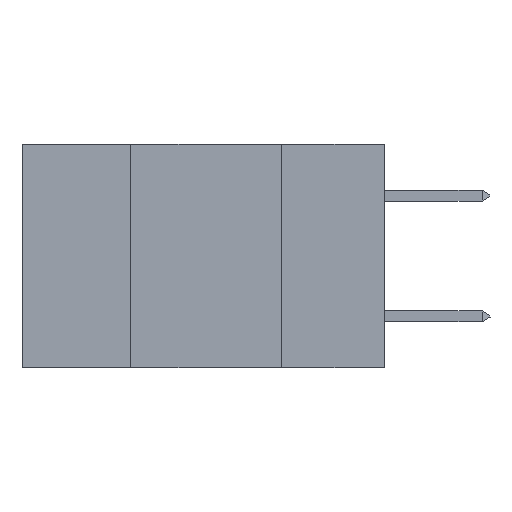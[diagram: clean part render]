
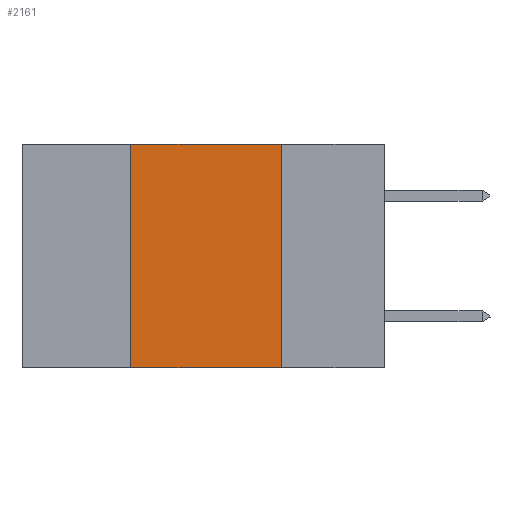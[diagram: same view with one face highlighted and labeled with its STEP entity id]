
A CAD part, left-side view. The second image highlights one B-rep face of the part: STEP entity #2161.
In plain terms, the highlighted planar face has unit normal (-1, 0, 0).
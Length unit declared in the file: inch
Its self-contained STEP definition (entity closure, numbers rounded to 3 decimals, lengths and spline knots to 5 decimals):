
#735 = VERTEX_POINT ( 'NONE', #7544 ) ;
#887 = CARTESIAN_POINT ( 'NONE',  ( 0., 0.42, -0.37 ) ) ;
#976 = VECTOR ( 'NONE', #5215, 39.37008 ) ;
#1231 = VERTEX_POINT ( 'NONE', #7557 ) ;
#1275 = VECTOR ( 'NONE', #4419, 39.37008 ) ;
#1786 = EDGE_LOOP ( 'NONE', ( #6654, #8103, #6742, #5730 ) ) ;
#2161 = ADVANCED_FACE ( 'NONE', ( #8982 ), #8652, .F. ) ;
#2275 = CARTESIAN_POINT ( 'NONE',  ( 0., 0.42, 0. ) ) ;
#2564 = EDGE_CURVE ( 'NONE', #8297, #735, #4637, .T. ) ;
#2744 = EDGE_CURVE ( 'NONE', #1231, #7260, #3077, .T. ) ;
#2819 = CARTESIAN_POINT ( 'NONE',  ( 0., 0.17, 0. ) ) ;
#2945 = DIRECTION ( 'NONE',  ( 0., 0., 1. ) ) ;
#3077 = LINE ( 'NONE', #4408, #1275 ) ;
#3910 = CARTESIAN_POINT ( 'NONE',  ( 0., 0.17, 0. ) ) ;
#4101 = CARTESIAN_POINT ( 'NONE',  ( 0., 0.6, -0.37 ) ) ;
#4186 = VECTOR ( 'NONE', #6700, 39.37008 ) ;
#4408 = CARTESIAN_POINT ( 'NONE',  ( 0., 0.6, 0. ) ) ;
#4419 = DIRECTION ( 'NONE',  ( 0., -1., 0. ) ) ;
#4572 = LINE ( 'NONE', #2275, #8159 ) ;
#4637 = LINE ( 'NONE', #4101, #4186 ) ;
#5215 = DIRECTION ( 'NONE',  ( 0., 0., -1. ) ) ;
#5413 = DIRECTION ( 'NONE',  ( 1., 0., 0. ) ) ;
#5577 = CARTESIAN_POINT ( 'NONE',  ( 0., 0.6, 0. ) ) ;
#5730 = ORIENTED_EDGE ( 'NONE', *, *, #2564, .T. ) ;
#5745 = EDGE_CURVE ( 'NONE', #7260, #735, #6426, .T. ) ;
#5927 = DIRECTION ( 'NONE',  ( 0., 0., -1. ) ) ;
#6426 = LINE ( 'NONE', #3910, #976 ) ;
#6654 = ORIENTED_EDGE ( 'NONE', *, *, #5745, .F. ) ;
#6700 = DIRECTION ( 'NONE',  ( 0., -1., 0. ) ) ;
#6742 = ORIENTED_EDGE ( 'NONE', *, *, #9050, .F. ) ;
#7260 = VERTEX_POINT ( 'NONE', #2819 ) ;
#7544 = CARTESIAN_POINT ( 'NONE',  ( 0., 0.17, -0.37 ) ) ;
#7557 = CARTESIAN_POINT ( 'NONE',  ( 0., 0.42, 0. ) ) ;
#8083 = AXIS2_PLACEMENT_3D ( 'NONE', #5577, #5413, #5927 ) ;
#8103 = ORIENTED_EDGE ( 'NONE', *, *, #2744, .F. ) ;
#8159 = VECTOR ( 'NONE', #2945, 39.37008 ) ;
#8297 = VERTEX_POINT ( 'NONE', #887 ) ;
#8652 = PLANE ( 'NONE',  #8083 ) ;
#8982 = FACE_OUTER_BOUND ( 'NONE', #1786, .T. ) ;
#9050 = EDGE_CURVE ( 'NONE', #8297, #1231, #4572, .T. ) ;
